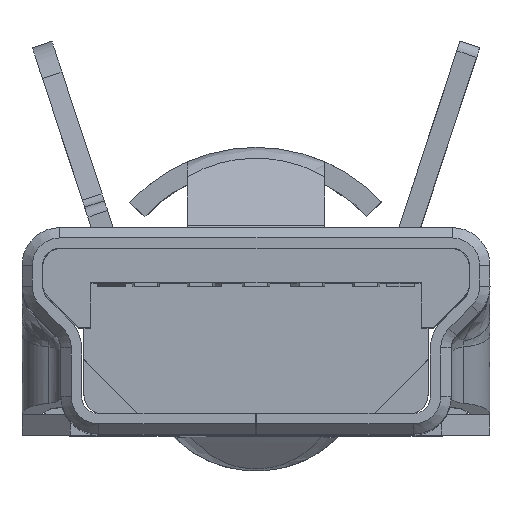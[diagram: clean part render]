
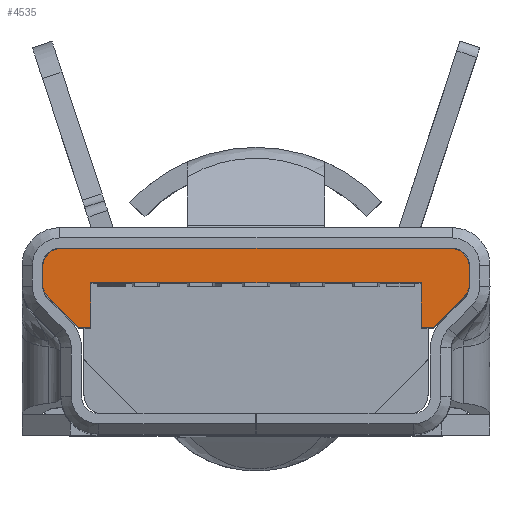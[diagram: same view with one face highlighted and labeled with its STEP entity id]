
A CAD part, top view. The second image highlights one B-rep face of the part: STEP entity #4535.
In plain terms, the highlighted planar face has unit normal (0, 0, 1).
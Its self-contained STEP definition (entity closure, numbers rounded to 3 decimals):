
#49 = ORIENTED_EDGE ( 'NONE', *, *, #12331, .T. ) ;
#76 = VECTOR ( 'NONE', #13207, 1000. ) ;
#81 = EDGE_CURVE ( 'NONE', #10846, #2278, #6975, .T. ) ;
#97 = CARTESIAN_POINT ( 'NONE',  ( 2.4, 0.8, 0. ) ) ;
#187 = DIRECTION ( 'NONE',  ( 1., 0., 0. ) ) ;
#255 = VECTOR ( 'NONE', #14352, 1000. ) ;
#554 = LINE ( 'NONE', #9157, #9041 ) ;
#581 = EDGE_CURVE ( 'NONE', #14870, #12370, #14607, .T. ) ;
#1169 = ORIENTED_EDGE ( 'NONE', *, *, #14228, .F. ) ;
#1368 = CARTESIAN_POINT ( 'NONE',  ( 3.1, 0.58, 0. ) ) ;
#1468 = LINE ( 'NONE', #13613, #9424 ) ;
#1553 = LINE ( 'NONE', #2765, #5688 ) ;
#1604 = VECTOR ( 'NONE', #11295, 1000. ) ;
#1973 = EDGE_CURVE ( 'NONE', #9996, #13303, #6216, .T. ) ;
#2120 = DIRECTION ( 'NONE',  ( 1., 0., 0. ) ) ;
#2148 = DIRECTION ( 'NONE',  ( 1., 0., 0. ) ) ;
#2207 = CARTESIAN_POINT ( 'NONE',  ( -3.1, 0.58, 0. ) ) ;
#2278 = VERTEX_POINT ( 'NONE', #12320 ) ;
#2554 = VERTEX_POINT ( 'NONE', #1368 ) ;
#2612 = CARTESIAN_POINT ( 'NONE',  ( -2.4, 1.45, 0. ) ) ;
#2628 = VERTEX_POINT ( 'NONE', #15291 ) ;
#2661 = CARTESIAN_POINT ( 'NONE',  ( 2.4, 1.125, 0. ) ) ;
#2765 = CARTESIAN_POINT ( 'NONE',  ( 3.1, 0.696, 0. ) ) ;
#3146 = ORIENTED_EDGE ( 'NONE', *, *, #8440, .F. ) ;
#3164 = CARTESIAN_POINT ( 'NONE',  ( 2.82, 0.813, 0. ) ) ;
#3321 = VERTEX_POINT ( 'NONE', #97 ) ;
#3814 = VERTEX_POINT ( 'NONE', #9792 ) ;
#3942 = DIRECTION ( 'NONE',  ( 1., 0., 0. ) ) ;
#4151 = EDGE_LOOP ( 'NONE', ( #13028, #49, #9943, #9498, #12483, #15038, #10595, #8587, #11824, #7218, #8001, #3146, #10830, #1169 ) ) ;
#4191 = EDGE_CURVE ( 'NONE', #10846, #3814, #5516, .T. ) ;
#4402 = DIRECTION ( 'NONE',  ( -1., 0., 0. ) ) ;
#4482 = DIRECTION ( 'NONE',  ( 0., 0., 1. ) ) ;
#4496 = AXIS2_PLACEMENT_3D ( 'NONE', #3164, #10410, #2120 ) ;
#4535 = ADVANCED_FACE ( 'NONE', ( #13945 ), #14984, .T. ) ;
#4669 = EDGE_CURVE ( 'NONE', #2628, #5519, #6533, .T. ) ;
#5081 = CARTESIAN_POINT ( 'NONE',  ( -3.224, 0.277, 0. ) ) ;
#5142 = DIRECTION ( 'NONE',  ( 0., 0., 1. ) ) ;
#5516 = CIRCLE ( 'NONE', #6019, 0.28 ) ;
#5519 = VERTEX_POINT ( 'NONE', #7493 ) ;
#5688 = VECTOR ( 'NONE', #9022, 1000. ) ;
#6019 = AXIS2_PLACEMENT_3D ( 'NONE', #8340, #4482, #13260 ) ;
#6069 = CARTESIAN_POINT ( 'NONE',  ( 0., 0.3, 0. ) ) ;
#6216 = LINE ( 'NONE', #6380, #1604 ) ;
#6294 = VECTOR ( 'NONE', #12951, 1000. ) ;
#6380 = CARTESIAN_POINT ( 'NONE',  ( 0., 1.45, 0. ) ) ;
#6533 = CIRCLE ( 'NONE', #4496, 0.28 ) ;
#6975 = LINE ( 'NONE', #8119, #6294 ) ;
#6998 = LINE ( 'NONE', #13291, #76 ) ;
#7173 = CARTESIAN_POINT ( 'NONE',  ( -3.1, 0.696, 0. ) ) ;
#7213 = CARTESIAN_POINT ( 'NONE',  ( -2.82, 0.58, 0. ) ) ;
#7218 = ORIENTED_EDGE ( 'NONE', *, *, #581, .T. ) ;
#7247 = EDGE_CURVE ( 'NONE', #12370, #2554, #10268, .T. ) ;
#7493 = CARTESIAN_POINT ( 'NONE',  ( 3.019, 1.01, 0. ) ) ;
#8001 = ORIENTED_EDGE ( 'NONE', *, *, #7247, .T. ) ;
#8119 = CARTESIAN_POINT ( 'NONE',  ( -2.801, 1.23, 0. ) ) ;
#8142 = CARTESIAN_POINT ( 'NONE',  ( 2.583, 1.45, 0. ) ) ;
#8303 = LINE ( 'NONE', #13216, #255 ) ;
#8340 = CARTESIAN_POINT ( 'NONE',  ( -2.82, 0.813, 0. ) ) ;
#8440 = EDGE_CURVE ( 'NONE', #2628, #2554, #1553, .T. ) ;
#8587 = ORIENTED_EDGE ( 'NONE', *, *, #14069, .F. ) ;
#8664 = DIRECTION ( 'NONE',  ( 0., 0., 1. ) ) ;
#8710 = AXIS2_PLACEMENT_3D ( 'NONE', #9807, #5142, #3942 ) ;
#8867 = DIRECTION ( 'NONE',  ( 0., 0., 1. ) ) ;
#8944 = EDGE_CURVE ( 'NONE', #3321, #12294, #554, .T. ) ;
#9022 = DIRECTION ( 'NONE',  ( 0., -1., 0. ) ) ;
#9041 = VECTOR ( 'NONE', #4402, 1000. ) ;
#9157 = CARTESIAN_POINT ( 'NONE',  ( 0., 0.8, 0. ) ) ;
#9360 = CARTESIAN_POINT ( 'NONE',  ( -3.019, 1.01, 0. ) ) ;
#9379 = CIRCLE ( 'NONE', #9886, 0.28 ) ;
#9424 = VECTOR ( 'NONE', #13537, 1000. ) ;
#9498 = ORIENTED_EDGE ( 'NONE', *, *, #9852, .T. ) ;
#9792 = CARTESIAN_POINT ( 'NONE',  ( -3.1, 0.813, 0. ) ) ;
#9807 = CARTESIAN_POINT ( 'NONE',  ( 2.82, 0.58, 0. ) ) ;
#9852 = EDGE_CURVE ( 'NONE', #12294, #10589, #8303, .T. ) ;
#9861 = VERTEX_POINT ( 'NONE', #2207 ) ;
#9886 = AXIS2_PLACEMENT_3D ( 'NONE', #7213, #8664, #13579 ) ;
#9943 = ORIENTED_EDGE ( 'NONE', *, *, #8944, .T. ) ;
#9996 = VERTEX_POINT ( 'NONE', #12239 ) ;
#10268 = CIRCLE ( 'NONE', #8710, 0.28 ) ;
#10410 = DIRECTION ( 'NONE',  ( 0., 0., 1. ) ) ;
#10589 = VERTEX_POINT ( 'NONE', #2612 ) ;
#10595 = ORIENTED_EDGE ( 'NONE', *, *, #4191, .T. ) ;
#10738 = DIRECTION ( 'NONE',  ( 0., 1., 0. ) ) ;
#10830 = ORIENTED_EDGE ( 'NONE', *, *, #4669, .T. ) ;
#10846 = VERTEX_POINT ( 'NONE', #9360 ) ;
#11025 = CARTESIAN_POINT ( 'NONE',  ( 2.82, 0.3, 0. ) ) ;
#11195 = VECTOR ( 'NONE', #10738, 1000. ) ;
#11295 = DIRECTION ( 'NONE',  ( 1., 0., 0. ) ) ;
#11405 = AXIS2_PLACEMENT_3D ( 'NONE', #5081, #8867, #187 ) ;
#11824 = ORIENTED_EDGE ( 'NONE', *, *, #12801, .T. ) ;
#11933 = VECTOR ( 'NONE', #14649, 1000. ) ;
#12011 = LINE ( 'NONE', #7173, #11195 ) ;
#12199 = VECTOR ( 'NONE', #2148, 1000. ) ;
#12239 = CARTESIAN_POINT ( 'NONE',  ( 2.4, 1.45, 0. ) ) ;
#12294 = VERTEX_POINT ( 'NONE', #15925 ) ;
#12320 = CARTESIAN_POINT ( 'NONE',  ( -2.583, 1.45, 0. ) ) ;
#12331 = EDGE_CURVE ( 'NONE', #9996, #3321, #12468, .T. ) ;
#12370 = VERTEX_POINT ( 'NONE', #11025 ) ;
#12468 = LINE ( 'NONE', #2661, #11933 ) ;
#12483 = ORIENTED_EDGE ( 'NONE', *, *, #15474, .F. ) ;
#12713 = CARTESIAN_POINT ( 'NONE',  ( -2.82, 0.3, 0. ) ) ;
#12801 = EDGE_CURVE ( 'NONE', #9861, #14870, #9379, .T. ) ;
#12951 = DIRECTION ( 'NONE',  ( 0.704, 0.71, 0. ) ) ;
#13028 = ORIENTED_EDGE ( 'NONE', *, *, #1973, .F. ) ;
#13207 = DIRECTION ( 'NONE',  ( 1., 0., 0. ) ) ;
#13216 = CARTESIAN_POINT ( 'NONE',  ( -2.4, 1.125, 0. ) ) ;
#13260 = DIRECTION ( 'NONE',  ( 1., 0., 0. ) ) ;
#13291 = CARTESIAN_POINT ( 'NONE',  ( 0., 1.45, 0. ) ) ;
#13303 = VERTEX_POINT ( 'NONE', #8142 ) ;
#13537 = DIRECTION ( 'NONE',  ( 0.704, -0.71, 0. ) ) ;
#13579 = DIRECTION ( 'NONE',  ( 1., 0., 0. ) ) ;
#13613 = CARTESIAN_POINT ( 'NONE',  ( 2.801, 1.23, 0. ) ) ;
#13945 = FACE_OUTER_BOUND ( 'NONE', #4151, .T. ) ;
#14069 = EDGE_CURVE ( 'NONE', #9861, #3814, #12011, .T. ) ;
#14228 = EDGE_CURVE ( 'NONE', #13303, #5519, #1468, .T. ) ;
#14352 = DIRECTION ( 'NONE',  ( 0., 1., 0. ) ) ;
#14607 = LINE ( 'NONE', #6069, #12199 ) ;
#14649 = DIRECTION ( 'NONE',  ( 0., -1., 0. ) ) ;
#14870 = VERTEX_POINT ( 'NONE', #12713 ) ;
#14984 = PLANE ( 'NONE',  #11405 ) ;
#15038 = ORIENTED_EDGE ( 'NONE', *, *, #81, .F. ) ;
#15291 = CARTESIAN_POINT ( 'NONE',  ( 3.1, 0.813, 0. ) ) ;
#15474 = EDGE_CURVE ( 'NONE', #2278, #10589, #6998, .T. ) ;
#15925 = CARTESIAN_POINT ( 'NONE',  ( -2.4, 0.8, 0. ) ) ;
